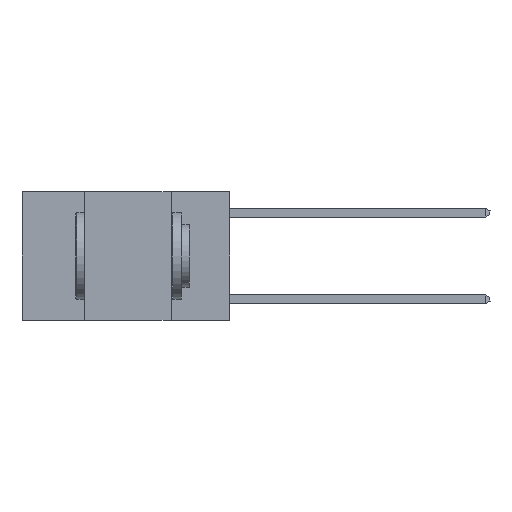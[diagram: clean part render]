
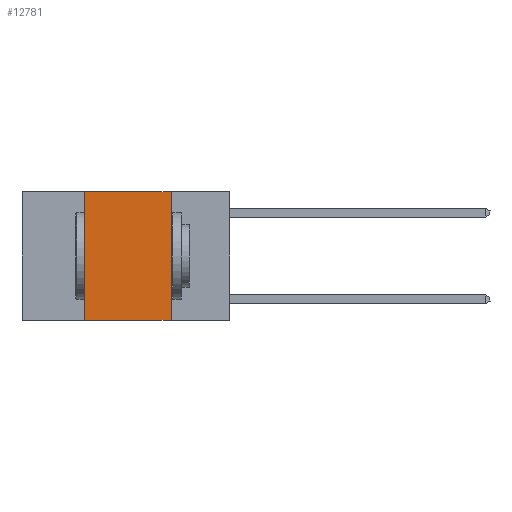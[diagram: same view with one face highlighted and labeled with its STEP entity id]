
A CAD part, left-side view. The second image highlights one B-rep face of the part: STEP entity #12781.
In plain terms, the highlighted planar face has unit normal (-1, 0, 0).
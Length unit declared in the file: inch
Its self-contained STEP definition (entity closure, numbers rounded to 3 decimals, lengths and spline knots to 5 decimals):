
#113 = EDGE_CURVE ( 'NONE', #6052, #6744, #2371, .T. ) ;
#778 = EDGE_CURVE ( 'NONE', #6744, #1109, #14938, .T. ) ;
#810 = ORIENTED_EDGE ( 'NONE', *, *, #778, .F. ) ;
#1109 = VERTEX_POINT ( 'NONE', #13584 ) ;
#1722 = EDGE_CURVE ( 'NONE', #1109, #4415, #13824, .T. ) ;
#2371 = LINE ( 'NONE', #3601, #8192 ) ;
#3023 = CARTESIAN_POINT ( 'NONE',  ( 0., 0.6, 0. ) ) ;
#3601 = CARTESIAN_POINT ( 'NONE',  ( 0., 0.42, 0. ) ) ;
#4415 = VERTEX_POINT ( 'NONE', #6854 ) ;
#4748 = CARTESIAN_POINT ( 'NONE',  ( 0., 0.42, 0. ) ) ;
#5647 = FACE_OUTER_BOUND ( 'NONE', #10483, .T. ) ;
#5694 = ORIENTED_EDGE ( 'NONE', *, *, #13620, .T. ) ;
#5915 = DIRECTION ( 'NONE',  ( 0., 0., 1. ) ) ;
#6052 = VERTEX_POINT ( 'NONE', #14989 ) ;
#6744 = VERTEX_POINT ( 'NONE', #4748 ) ;
#6854 = CARTESIAN_POINT ( 'NONE',  ( 0., 0.17, -0.37 ) ) ;
#7709 = DIRECTION ( 'NONE',  ( 0., -1., 0. ) ) ;
#7837 = DIRECTION ( 'NONE',  ( 0., 0., -1. ) ) ;
#8192 = VECTOR ( 'NONE', #5915, 39.37008 ) ;
#9110 = DIRECTION ( 'NONE',  ( 0., 0., -1. ) ) ;
#9259 = CARTESIAN_POINT ( 'NONE',  ( 0., 0.6, 0. ) ) ;
#9678 = VECTOR ( 'NONE', #7709, 39.37008 ) ;
#9711 = VECTOR ( 'NONE', #7837, 39.37008 ) ;
#10483 = EDGE_LOOP ( 'NONE', ( #12851, #810, #11770, #5694 ) ) ;
#10493 = DIRECTION ( 'NONE',  ( 1., 0., 0. ) ) ;
#10828 = CARTESIAN_POINT ( 'NONE',  ( 0., 0.6, -0.37 ) ) ;
#11435 = PLANE ( 'NONE',  #11533 ) ;
#11533 = AXIS2_PLACEMENT_3D ( 'NONE', #9259, #10493, #9110 ) ;
#11538 = CARTESIAN_POINT ( 'NONE',  ( 0., 0.17, 0. ) ) ;
#11542 = VECTOR ( 'NONE', #14279, 39.37008 ) ;
#11770 = ORIENTED_EDGE ( 'NONE', *, *, #113, .F. ) ;
#12058 = LINE ( 'NONE', #10828, #11542 ) ;
#12781 = ADVANCED_FACE ( 'NONE', ( #5647 ), #11435, .F. ) ;
#12851 = ORIENTED_EDGE ( 'NONE', *, *, #1722, .F. ) ;
#13584 = CARTESIAN_POINT ( 'NONE',  ( 0., 0.17, 0. ) ) ;
#13620 = EDGE_CURVE ( 'NONE', #6052, #4415, #12058, .T. ) ;
#13824 = LINE ( 'NONE', #11538, #9711 ) ;
#14279 = DIRECTION ( 'NONE',  ( 0., -1., 0. ) ) ;
#14938 = LINE ( 'NONE', #3023, #9678 ) ;
#14989 = CARTESIAN_POINT ( 'NONE',  ( 0., 0.42, -0.37 ) ) ;
